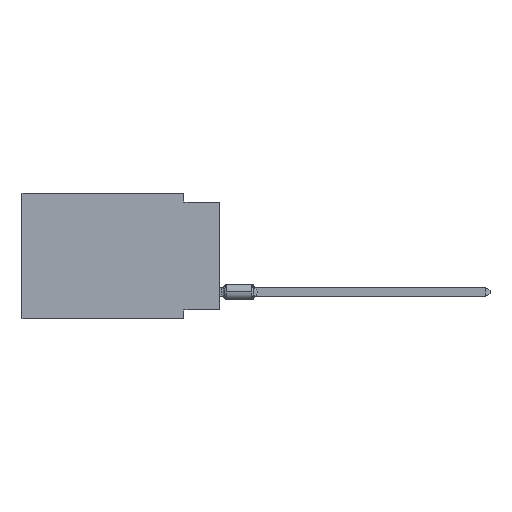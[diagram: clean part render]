
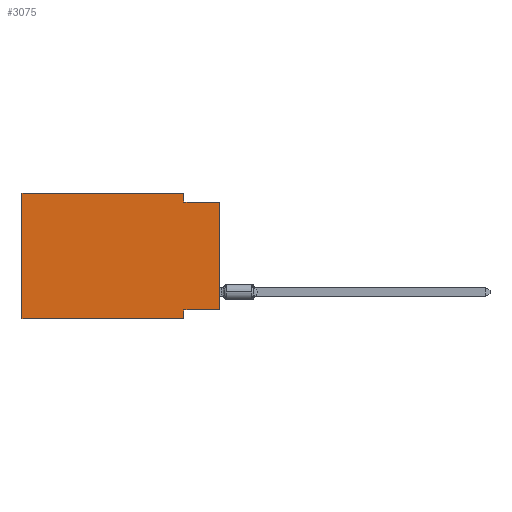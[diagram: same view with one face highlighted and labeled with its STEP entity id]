
A CAD part, left-side view. The second image highlights one B-rep face of the part: STEP entity #3075.
In plain terms, the highlighted planar face has unit normal (-1, 0, 0).
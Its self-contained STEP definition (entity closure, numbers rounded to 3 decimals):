
#690 = EDGE_CURVE ( 'NONE', #35220, #38487, #26609, .T. ) ;
#1529 = VECTOR ( 'NONE', #13992, 1000. ) ;
#1874 = DIRECTION ( 'NONE',  ( 0., 0., -1. ) ) ;
#2999 = CARTESIAN_POINT ( 'NONE',  ( 0., 0., 0. ) ) ;
#3075 = ADVANCED_FACE ( 'NONE', ( #28745 ), #26157, .F. ) ;
#3202 = CARTESIAN_POINT ( 'NONE',  ( 0., 13.97, 0. ) ) ;
#3870 = VERTEX_POINT ( 'NONE', #5124 ) ;
#4261 = VECTOR ( 'NONE', #11700, 1000. ) ;
#4319 = VECTOR ( 'NONE', #29383, 1000. ) ;
#4632 = LINE ( 'NONE', #10355, #29347 ) ;
#4809 = EDGE_CURVE ( 'NONE', #38487, #23795, #12082, .T. ) ;
#5124 = CARTESIAN_POINT ( 'NONE',  ( 0., 2.54, -0.635 ) ) ;
#6331 = DIRECTION ( 'NONE',  ( 0., 0., 1. ) ) ;
#6683 = ORIENTED_EDGE ( 'NONE', *, *, #21994, .T. ) ;
#6730 = CARTESIAN_POINT ( 'NONE',  ( 0., 2.54, -8.89 ) ) ;
#6933 = VERTEX_POINT ( 'NONE', #27622 ) ;
#7175 = CARTESIAN_POINT ( 'NONE',  ( 0., 0., -0.635 ) ) ;
#7874 = ORIENTED_EDGE ( 'NONE', *, *, #690, .F. ) ;
#8565 = DIRECTION ( 'NONE',  ( 0., 0., -1. ) ) ;
#8956 = LINE ( 'NONE', #11938, #19699 ) ;
#10355 = CARTESIAN_POINT ( 'NONE',  ( 0., 2.54, 0. ) ) ;
#10421 = VECTOR ( 'NONE', #21555, 1000. ) ;
#10832 = LINE ( 'NONE', #19546, #1529 ) ;
#10990 = CARTESIAN_POINT ( 'NONE',  ( 0., 13.97, 0. ) ) ;
#11090 = ORIENTED_EDGE ( 'NONE', *, *, #11569, .F. ) ;
#11150 = CARTESIAN_POINT ( 'NONE',  ( 0., 13.97, 0. ) ) ;
#11508 = EDGE_LOOP ( 'NONE', ( #6683, #19790, #36088, #32039, #7874, #29130, #34035, #11090 ) ) ;
#11569 = EDGE_CURVE ( 'NONE', #20677, #15469, #10832, .T. ) ;
#11700 = DIRECTION ( 'NONE',  ( 0., -1., 0. ) ) ;
#11938 = CARTESIAN_POINT ( 'NONE',  ( 0., 13.97, -8.89 ) ) ;
#12082 = LINE ( 'NONE', #3202, #4261 ) ;
#12295 = EDGE_CURVE ( 'NONE', #3870, #13462, #19454, .T. ) ;
#13462 = VERTEX_POINT ( 'NONE', #37229 ) ;
#13992 = DIRECTION ( 'NONE',  ( 0., 1., 0. ) ) ;
#14517 = DIRECTION ( 'NONE',  ( 0., -1., 0. ) ) ;
#15469 = VERTEX_POINT ( 'NONE', #37484 ) ;
#15661 = VECTOR ( 'NONE', #37806, 1000. ) ;
#15781 = CARTESIAN_POINT ( 'NONE',  ( 0., 2.54, 0. ) ) ;
#17584 = CARTESIAN_POINT ( 'NONE',  ( 0., 13.97, -8.89 ) ) ;
#19454 = LINE ( 'NONE', #7175, #15661 ) ;
#19546 = CARTESIAN_POINT ( 'NONE',  ( 0., 0., -8.255 ) ) ;
#19699 = VECTOR ( 'NONE', #14517, 1000. ) ;
#19790 = ORIENTED_EDGE ( 'NONE', *, *, #12295, .F. ) ;
#20677 = VERTEX_POINT ( 'NONE', #34072 ) ;
#21555 = DIRECTION ( 'NONE',  ( 0., 0., -1. ) ) ;
#21743 = LINE ( 'NONE', #6730, #10421 ) ;
#21994 = EDGE_CURVE ( 'NONE', #20677, #13462, #38929, .T. ) ;
#23517 = CARTESIAN_POINT ( 'NONE',  ( 0., 13.97, 0. ) ) ;
#23795 = VERTEX_POINT ( 'NONE', #15781 ) ;
#24402 = EDGE_CURVE ( 'NONE', #35220, #6933, #8956, .T. ) ;
#24658 = AXIS2_PLACEMENT_3D ( 'NONE', #11150, #35635, #8565 ) ;
#25495 = VECTOR ( 'NONE', #6331, 1000. ) ;
#26157 = PLANE ( 'NONE',  #24658 ) ;
#26609 = LINE ( 'NONE', #10990, #4319 ) ;
#27622 = CARTESIAN_POINT ( 'NONE',  ( 0., 2.54, -8.89 ) ) ;
#28745 = FACE_OUTER_BOUND ( 'NONE', #11508, .T. ) ;
#29130 = ORIENTED_EDGE ( 'NONE', *, *, #24402, .T. ) ;
#29347 = VECTOR ( 'NONE', #1874, 1000. ) ;
#29383 = DIRECTION ( 'NONE',  ( 0., 0., 1. ) ) ;
#32039 = ORIENTED_EDGE ( 'NONE', *, *, #4809, .F. ) ;
#33285 = EDGE_CURVE ( 'NONE', #23795, #3870, #4632, .T. ) ;
#33713 = EDGE_CURVE ( 'NONE', #15469, #6933, #21743, .T. ) ;
#34035 = ORIENTED_EDGE ( 'NONE', *, *, #33713, .F. ) ;
#34072 = CARTESIAN_POINT ( 'NONE',  ( 0., 0., -8.255 ) ) ;
#35220 = VERTEX_POINT ( 'NONE', #17584 ) ;
#35635 = DIRECTION ( 'NONE',  ( 1., 0., 0. ) ) ;
#36088 = ORIENTED_EDGE ( 'NONE', *, *, #33285, .F. ) ;
#37229 = CARTESIAN_POINT ( 'NONE',  ( 0., 0., -0.635 ) ) ;
#37484 = CARTESIAN_POINT ( 'NONE',  ( 0., 2.54, -8.255 ) ) ;
#37806 = DIRECTION ( 'NONE',  ( 0., -1., 0. ) ) ;
#38487 = VERTEX_POINT ( 'NONE', #23517 ) ;
#38929 = LINE ( 'NONE', #2999, #25495 ) ;
